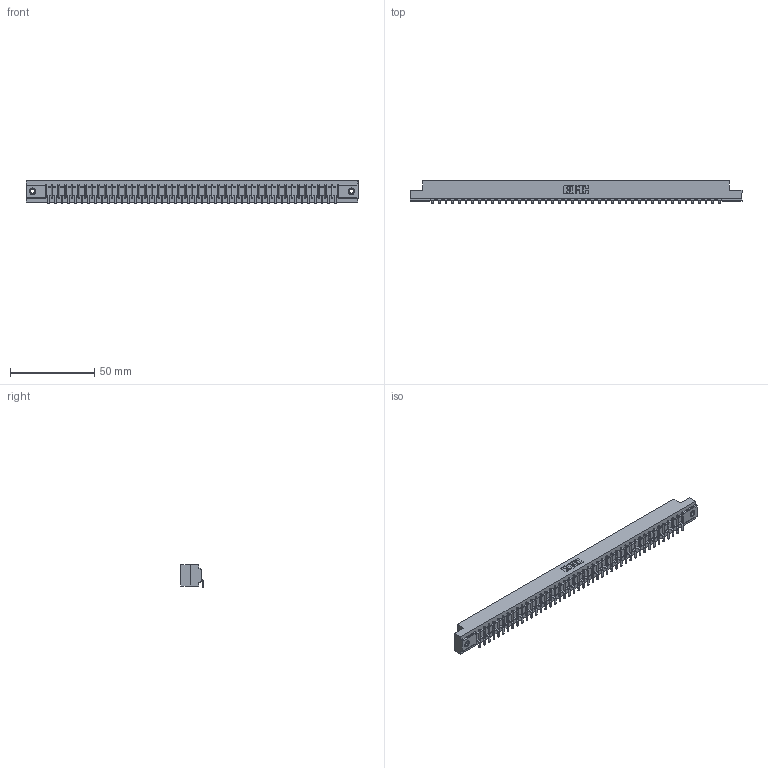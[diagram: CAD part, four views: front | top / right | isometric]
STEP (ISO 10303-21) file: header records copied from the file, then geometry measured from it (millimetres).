
FILE_DESCRIPTION (( 'STEP AP203' ), '1' );
FILE_NAME ('307-044-553-107.STEP', '2018-08-06T01:56:49', ( '' ), ( '' ), 'SwSTEP 2.0', 'SolidWorks 2016', '' );
FILE_SCHEMA (( 'CONFIG_CONTROL_DESIGN' ));
Length unit declared in the file: inch
Products named in the file (4): 307 Part_.156 Dia Mounting Holes; 307-290-002_553; 345-250-001_345-250-005-103; 307-044-553-107
Assembly tree (47 placements, depth 2):
  307-044-553-107
    307 Part_.156 Dia Mounting Holes
    307-290-002_553  x44
    345-250-001_345-250-005-103  x2
Bounding box: 197.36 x 13.32 x 13.5 mm (x, y, z)
Volume: 21121 mm3; surface area: 26625.6 mm2
Topology: 47 solids, 47 shells, 3655 faces, 11195 edges, 7334 vertices
Faces by surface type: plane 2170, cylinder 1379, sphere 90, cone 12, torus 4
Entity records: 39513 total; most frequent: CARTESIAN_POINT 6647, ORIENTED_EDGE 6630, DIRECTION 6467, EDGE_CURVE 3315, LINE 2539, VECTOR 2539, VERTEX_POINT 2144, AXIS2_PLACEMENT_3D 1964
